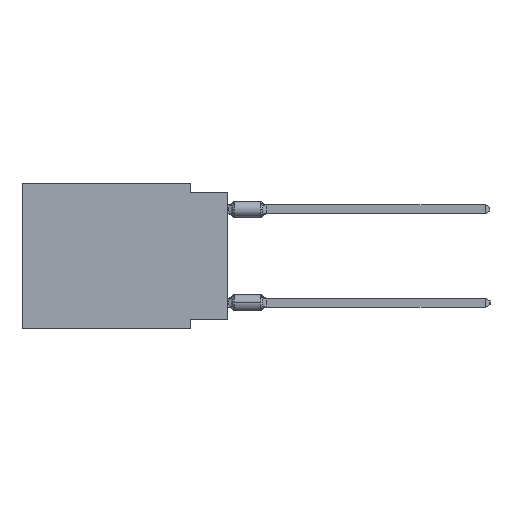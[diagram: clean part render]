
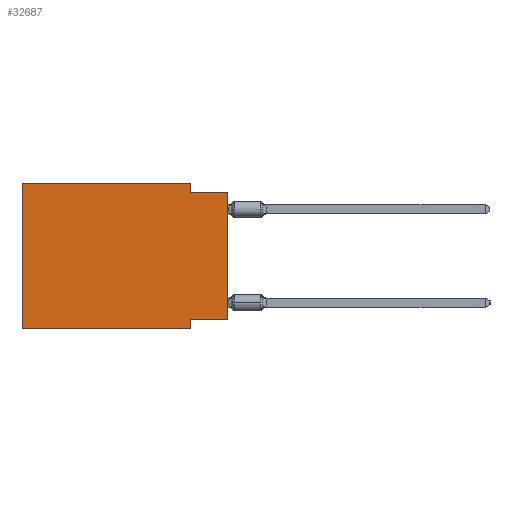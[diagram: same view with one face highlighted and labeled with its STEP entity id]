
A CAD part, left-side view. The second image highlights one B-rep face of the part: STEP entity #32687.
In plain terms, the highlighted planar face has unit normal (-1, 0, 0).
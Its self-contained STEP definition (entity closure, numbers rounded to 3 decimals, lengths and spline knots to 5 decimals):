
#1130 = CARTESIAN_POINT ( 'NONE',  ( 0., 0.1, -0.39 ) ) ;
#1672 = VERTEX_POINT ( 'NONE', #11177 ) ;
#1997 = ORIENTED_EDGE ( 'NONE', *, *, #51106, .F. ) ;
#3904 = VECTOR ( 'NONE', #10450, 39.37008 ) ;
#4726 = EDGE_CURVE ( 'NONE', #12547, #44979, #12147, .T. ) ;
#6046 = CARTESIAN_POINT ( 'NONE',  ( 0., 0., 0. ) ) ;
#6482 = VECTOR ( 'NONE', #55164, 39.37008 ) ;
#7941 = CARTESIAN_POINT ( 'NONE',  ( 0., 0.55, 0. ) ) ;
#10450 = DIRECTION ( 'NONE',  ( 0., 0., -1. ) ) ;
#11177 = CARTESIAN_POINT ( 'NONE',  ( 0., 0.1, -0.025 ) ) ;
#11400 = FACE_OUTER_BOUND ( 'NONE', #13109, .T. ) ;
#11813 = VECTOR ( 'NONE', #56037, 39.37008 ) ;
#12147 = LINE ( 'NONE', #7941, #31389 ) ;
#12547 = VERTEX_POINT ( 'NONE', #28257 ) ;
#13109 = EDGE_LOOP ( 'NONE', ( #62719, #34938, #52921, #1997, #51575, #47751, #26411, #57182 ) ) ;
#15799 = CARTESIAN_POINT ( 'NONE',  ( 0., 0.55, 0. ) ) ;
#16337 = DIRECTION ( 'NONE',  ( 0., 0., 1. ) ) ;
#16579 = CARTESIAN_POINT ( 'NONE',  ( 0., 0.1, 0. ) ) ;
#17520 = DIRECTION ( 'NONE',  ( 0., -1., 0. ) ) ;
#18687 = VECTOR ( 'NONE', #17520, 39.37008 ) ;
#19514 = VECTOR ( 'NONE', #33285, 39.37008 ) ;
#22094 = CARTESIAN_POINT ( 'NONE',  ( 0., 0.1, -0.39 ) ) ;
#22965 = LINE ( 'NONE', #16579, #11813 ) ;
#23277 = LINE ( 'NONE', #48283, #41046 ) ;
#23874 = VERTEX_POINT ( 'NONE', #45127 ) ;
#25682 = CARTESIAN_POINT ( 'NONE',  ( 0., 0., -0.025 ) ) ;
#25864 = PLANE ( 'NONE',  #28623 ) ;
#25957 = LINE ( 'NONE', #6046, #6482 ) ;
#26295 = EDGE_CURVE ( 'NONE', #57699, #1672, #22965, .T. ) ;
#26411 = ORIENTED_EDGE ( 'NONE', *, *, #31580, .F. ) ;
#28257 = CARTESIAN_POINT ( 'NONE',  ( 0., 0.55, -0.39 ) ) ;
#28434 = DIRECTION ( 'NONE',  ( 0., 1., 0. ) ) ;
#28623 = AXIS2_PLACEMENT_3D ( 'NONE', #40623, #35797, #40935 ) ;
#29097 = VECTOR ( 'NONE', #28434, 39.37008 ) ;
#31389 = VECTOR ( 'NONE', #16337, 39.37008 ) ;
#31580 = EDGE_CURVE ( 'NONE', #23874, #45283, #39662, .T. ) ;
#32687 = ADVANCED_FACE ( 'NONE', ( #11400 ), #25864, .F. ) ;
#32925 = CARTESIAN_POINT ( 'NONE',  ( 0., 0.55, 0. ) ) ;
#33285 = DIRECTION ( 'NONE',  ( 0., -1., 0. ) ) ;
#33533 = DIRECTION ( 'NONE',  ( 0., -1., 0. ) ) ;
#34032 = EDGE_CURVE ( 'NONE', #1672, #36640, #48684, .T. ) ;
#34343 = EDGE_CURVE ( 'NONE', #12547, #45283, #23277, .T. ) ;
#34938 = ORIENTED_EDGE ( 'NONE', *, *, #34032, .F. ) ;
#35797 = DIRECTION ( 'NONE',  ( 1., 0., 0. ) ) ;
#36640 = VERTEX_POINT ( 'NONE', #25682 ) ;
#39662 = LINE ( 'NONE', #1130, #3904 ) ;
#40623 = CARTESIAN_POINT ( 'NONE',  ( 0., 0.55, 0. ) ) ;
#40935 = DIRECTION ( 'NONE',  ( 0., 0., -1. ) ) ;
#41046 = VECTOR ( 'NONE', #33533, 39.37008 ) ;
#44475 = LINE ( 'NONE', #59224, #29097 ) ;
#44979 = VERTEX_POINT ( 'NONE', #15799 ) ;
#45127 = CARTESIAN_POINT ( 'NONE',  ( 0., 0.1, -0.365 ) ) ;
#45283 = VERTEX_POINT ( 'NONE', #22094 ) ;
#47751 = ORIENTED_EDGE ( 'NONE', *, *, #34343, .T. ) ;
#48283 = CARTESIAN_POINT ( 'NONE',  ( 0., 0.55, -0.39 ) ) ;
#48684 = LINE ( 'NONE', #58947, #19514 ) ;
#51106 = EDGE_CURVE ( 'NONE', #44979, #57699, #56042, .T. ) ;
#51575 = ORIENTED_EDGE ( 'NONE', *, *, #4726, .F. ) ;
#52469 = EDGE_CURVE ( 'NONE', #56608, #23874, #44475, .T. ) ;
#52921 = ORIENTED_EDGE ( 'NONE', *, *, #26295, .F. ) ;
#53971 = EDGE_CURVE ( 'NONE', #56608, #36640, #25957, .T. ) ;
#55164 = DIRECTION ( 'NONE',  ( 0., 0., 1. ) ) ;
#56037 = DIRECTION ( 'NONE',  ( 0., 0., -1. ) ) ;
#56042 = LINE ( 'NONE', #32925, #18687 ) ;
#56188 = CARTESIAN_POINT ( 'NONE',  ( 0., 0., -0.365 ) ) ;
#56608 = VERTEX_POINT ( 'NONE', #56188 ) ;
#57182 = ORIENTED_EDGE ( 'NONE', *, *, #52469, .F. ) ;
#57699 = VERTEX_POINT ( 'NONE', #60205 ) ;
#58947 = CARTESIAN_POINT ( 'NONE',  ( 0., 0., -0.025 ) ) ;
#59224 = CARTESIAN_POINT ( 'NONE',  ( 0., 0., -0.365 ) ) ;
#60205 = CARTESIAN_POINT ( 'NONE',  ( 0., 0.1, 0. ) ) ;
#62719 = ORIENTED_EDGE ( 'NONE', *, *, #53971, .T. ) ;
